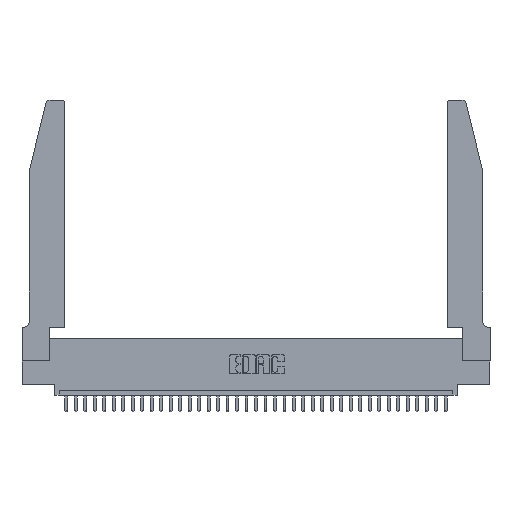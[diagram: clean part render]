
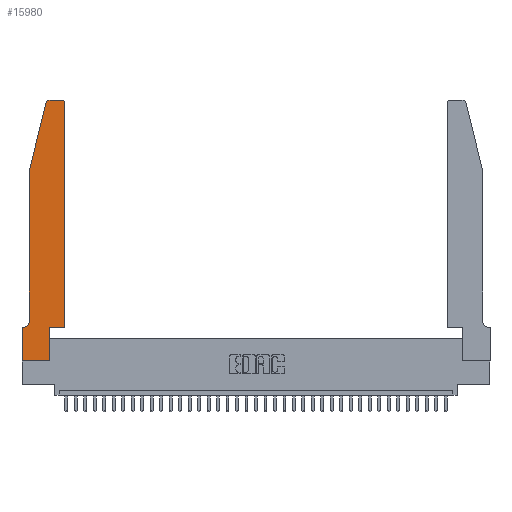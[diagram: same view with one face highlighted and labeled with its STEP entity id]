
A CAD part, top view. The second image highlights one B-rep face of the part: STEP entity #15980.
In plain terms, the highlighted planar face has unit normal (0, 0, 1).
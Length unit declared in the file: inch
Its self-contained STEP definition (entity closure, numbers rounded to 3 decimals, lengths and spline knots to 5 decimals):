
#840 = DIRECTION ( 'NONE',  ( -1., 0., 0. ) ) ;
#871 = CARTESIAN_POINT ( 'NONE',  ( 0.284, 2.75, 0.37 ) ) ;
#1230 = ORIENTED_EDGE ( 'NONE', *, *, #32173, .T. ) ;
#1427 = VERTEX_POINT ( 'NONE', #27715 ) ;
#2090 = CARTESIAN_POINT ( 'NONE',  ( 0.4505, 0.35, 0.37 ) ) ;
#3076 = CARTESIAN_POINT ( 'NONE',  ( 0.0055, 0.42, 0.37 ) ) ;
#4383 = VERTEX_POINT ( 'NONE', #15943 ) ;
#4503 = DIRECTION ( 'NONE',  ( 1., 0., 0. ) ) ;
#4687 = LINE ( 'NONE', #16486, #33334 ) ;
#4702 = ORIENTED_EDGE ( 'NONE', *, *, #18146, .T. ) ;
#4914 = AXIS2_PLACEMENT_3D ( 'NONE', #3076, #22561, #28488 ) ;
#5058 = EDGE_CURVE ( 'NONE', #27906, #16165, #9597, .T. ) ;
#5268 = LINE ( 'NONE', #2090, #16555 ) ;
#5403 = CIRCLE ( 'NONE', #4914, 0.07 ) ;
#5638 = VECTOR ( 'NONE', #17413, 39.37008 ) ;
#6260 = LINE ( 'NONE', #23239, #8865 ) ;
#6495 = LINE ( 'NONE', #22883, #5638 ) ;
#6555 = DIRECTION ( 'NONE',  ( 1., 0., 0. ) ) ;
#7196 = CARTESIAN_POINT ( 'NONE',  ( 0.4205, 2.75, 0.37 ) ) ;
#7403 = PLANE ( 'NONE',  #30499 ) ;
#7445 = ORIENTED_EDGE ( 'NONE', *, *, #12350, .T. ) ;
#7662 = VERTEX_POINT ( 'NONE', #29820 ) ;
#7782 = ORIENTED_EDGE ( 'NONE', *, *, #34528, .T. ) ;
#7879 = VECTOR ( 'NONE', #33691, 39.37008 ) ;
#8865 = VECTOR ( 'NONE', #6555, 39.37008 ) ;
#9317 = EDGE_CURVE ( 'NONE', #4383, #7662, #17174, .T. ) ;
#9574 = CARTESIAN_POINT ( 'NONE',  ( 0.0055, 0.35, 0.37 ) ) ;
#9597 = LINE ( 'NONE', #35390, #7879 ) ;
#9817 = VERTEX_POINT ( 'NONE', #871 ) ;
#9999 = CARTESIAN_POINT ( 'NONE',  ( 0., 0., 0.37 ) ) ;
#10137 = ORIENTED_EDGE ( 'NONE', *, *, #10937, .T. ) ;
#10937 = EDGE_CURVE ( 'NONE', #16165, #4383, #6260, .T. ) ;
#11012 = ORIENTED_EDGE ( 'NONE', *, *, #33679, .T. ) ;
#11957 = FACE_OUTER_BOUND ( 'NONE', #24334, .T. ) ;
#12350 = EDGE_CURVE ( 'NONE', #7662, #16764, #27821, .T. ) ;
#13216 = ORIENTED_EDGE ( 'NONE', *, *, #31931, .T. ) ;
#13532 = CARTESIAN_POINT ( 'NONE',  ( 0.0755, 2., 0.37 ) ) ;
#13901 = EDGE_CURVE ( 'NONE', #17185, #27906, #14756, .T. ) ;
#14583 = CARTESIAN_POINT ( 'NONE',  ( 0.25487, 2.72718, 0.37 ) ) ;
#14746 = ORIENTED_EDGE ( 'NONE', *, *, #25231, .T. ) ;
#14756 = LINE ( 'NONE', #22865, #15231 ) ;
#14803 = CARTESIAN_POINT ( 'NONE',  ( 0.4205, 2.72, 0.37 ) ) ;
#15104 = ORIENTED_EDGE ( 'NONE', *, *, #31020, .T. ) ;
#15231 = VECTOR ( 'NONE', #840, 39.37008 ) ;
#15746 = VERTEX_POINT ( 'NONE', #17198 ) ;
#15749 = CARTESIAN_POINT ( 'NONE',  ( 0.284, 2.72, 0.37 ) ) ;
#15814 = DIRECTION ( 'NONE',  ( 0., 0., 1. ) ) ;
#15943 = CARTESIAN_POINT ( 'NONE',  ( 0.2865, 0., 0.37 ) ) ;
#15980 = ADVANCED_FACE ( 'NONE', ( #11957 ), #7403, .T. ) ;
#16153 = DIRECTION ( 'NONE',  ( -0.239, -0.971, 0. ) ) ;
#16165 = VERTEX_POINT ( 'NONE', #9999 ) ;
#16358 = VECTOR ( 'NONE', #26102, 39.37008 ) ;
#16486 = CARTESIAN_POINT ( 'NONE',  ( 0.0755, 2., 0.37 ) ) ;
#16555 = VECTOR ( 'NONE', #32729, 39.37008 ) ;
#16764 = VERTEX_POINT ( 'NONE', #28724 ) ;
#17174 = LINE ( 'NONE', #26831, #16358 ) ;
#17185 = VERTEX_POINT ( 'NONE', #9574 ) ;
#17198 = CARTESIAN_POINT ( 'NONE',  ( 0.0755, 0.42, 0.37 ) ) ;
#17413 = DIRECTION ( 'NONE',  ( -1., 0., 0. ) ) ;
#17775 = DIRECTION ( 'NONE',  ( 1., 0., 0. ) ) ;
#18146 = EDGE_CURVE ( 'NONE', #16764, #21705, #5268, .T. ) ;
#21705 = VERTEX_POINT ( 'NONE', #23397 ) ;
#22561 = DIRECTION ( 'NONE',  ( 0., 0., -1. ) ) ;
#22865 = CARTESIAN_POINT ( 'NONE',  ( 0.0755, 0.35, 0.37 ) ) ;
#22883 = CARTESIAN_POINT ( 'NONE',  ( 0.2605, 2.75, 0.37 ) ) ;
#23239 = CARTESIAN_POINT ( 'NONE',  ( 0., 0., 0.37 ) ) ;
#23397 = CARTESIAN_POINT ( 'NONE',  ( 0.4505, 2.72, 0.37 ) ) ;
#24111 = VERTEX_POINT ( 'NONE', #14583 ) ;
#24334 = EDGE_LOOP ( 'NONE', ( #14746, #7782, #1230, #15104, #11012, #33873, #26654, #10137, #35803, #7445, #4702, #13216 ) ) ;
#24626 = CARTESIAN_POINT ( 'NONE',  ( 0.4505, 0.35, 0.37 ) ) ;
#25231 = EDGE_CURVE ( 'NONE', #30939, #9817, #6495, .T. ) ;
#25447 = DIRECTION ( 'NONE',  ( 1., 0., 0. ) ) ;
#26102 = DIRECTION ( 'NONE',  ( 0., 1., 0. ) ) ;
#26475 = LINE ( 'NONE', #13532, #27347 ) ;
#26654 = ORIENTED_EDGE ( 'NONE', *, *, #5058, .T. ) ;
#26831 = CARTESIAN_POINT ( 'NONE',  ( 0.2865, 0.35, 0.37 ) ) ;
#27347 = VECTOR ( 'NONE', #35827, 39.37008 ) ;
#27715 = CARTESIAN_POINT ( 'NONE',  ( 0.0755, 2., 0.37 ) ) ;
#27821 = LINE ( 'NONE', #24626, #30829 ) ;
#27906 = VERTEX_POINT ( 'NONE', #27966 ) ;
#27966 = CARTESIAN_POINT ( 'NONE',  ( 0., 0.35, 0.37 ) ) ;
#28488 = DIRECTION ( 'NONE',  ( -1., 0., 0. ) ) ;
#28724 = CARTESIAN_POINT ( 'NONE',  ( 0.4505, 0.35, 0.37 ) ) ;
#29413 = DIRECTION ( 'NONE',  ( 1., 0., 0. ) ) ;
#29666 = DIRECTION ( 'NONE',  ( 0., 0., 1. ) ) ;
#29730 = CARTESIAN_POINT ( 'NONE',  ( 0., 0.35, 0.37 ) ) ;
#29820 = CARTESIAN_POINT ( 'NONE',  ( 0.2865, 0.35, 0.37 ) ) ;
#29861 = CIRCLE ( 'NONE', #32110, 0.03 ) ;
#30499 = AXIS2_PLACEMENT_3D ( 'NONE', #29730, #15814, #4503 ) ;
#30829 = VECTOR ( 'NONE', #17775, 39.37008 ) ;
#30939 = VERTEX_POINT ( 'NONE', #7196 ) ;
#31020 = EDGE_CURVE ( 'NONE', #1427, #15746, #26475, .T. ) ;
#31407 = DIRECTION ( 'NONE',  ( 0., 0., 1. ) ) ;
#31931 = EDGE_CURVE ( 'NONE', #21705, #30939, #29861, .T. ) ;
#32110 = AXIS2_PLACEMENT_3D ( 'NONE', #14803, #31407, #25447 ) ;
#32173 = EDGE_CURVE ( 'NONE', #24111, #1427, #4687, .T. ) ;
#32729 = DIRECTION ( 'NONE',  ( 0., 1., 0. ) ) ;
#33334 = VECTOR ( 'NONE', #16153, 39.37008 ) ;
#33679 = EDGE_CURVE ( 'NONE', #15746, #17185, #5403, .T. ) ;
#33691 = DIRECTION ( 'NONE',  ( 0., -1., 0. ) ) ;
#33873 = ORIENTED_EDGE ( 'NONE', *, *, #13901, .T. ) ;
#34528 = EDGE_CURVE ( 'NONE', #9817, #24111, #34966, .T. ) ;
#34966 = CIRCLE ( 'NONE', #35158, 0.03 ) ;
#35158 = AXIS2_PLACEMENT_3D ( 'NONE', #15749, #29666, #29413 ) ;
#35390 = CARTESIAN_POINT ( 'NONE',  ( 0., 0., 0.37 ) ) ;
#35803 = ORIENTED_EDGE ( 'NONE', *, *, #9317, .T. ) ;
#35827 = DIRECTION ( 'NONE',  ( 0., -1., 0. ) ) ;
